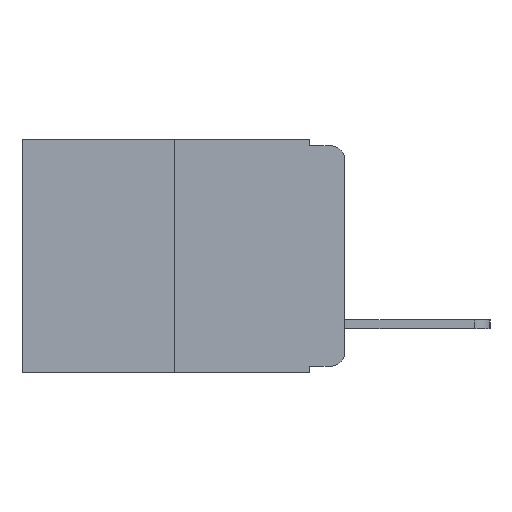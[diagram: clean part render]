
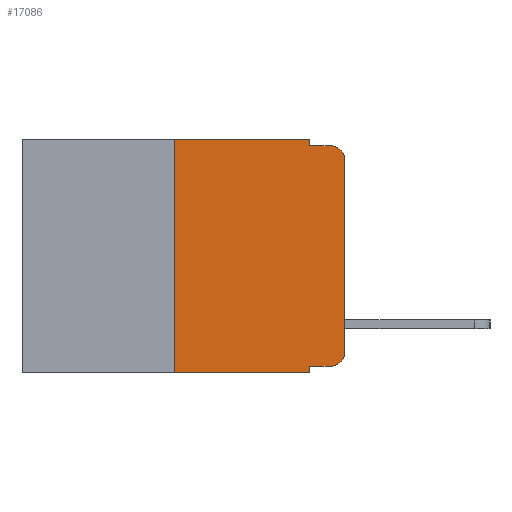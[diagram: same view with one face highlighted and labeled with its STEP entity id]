
A CAD part, left-side view. The second image highlights one B-rep face of the part: STEP entity #17086.
In plain terms, the highlighted planar face has unit normal (-1, 0, 0).
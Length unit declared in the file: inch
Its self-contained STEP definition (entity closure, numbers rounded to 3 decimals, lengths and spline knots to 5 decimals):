
#43 = DIRECTION ( 'NONE',  ( 0., 0., -1. ) ) ;
#70 = DIRECTION ( 'NONE',  ( 0., 0., -1. ) ) ;
#181 = CARTESIAN_POINT ( 'NONE',  ( 0., 0.051, -0.333 ) ) ;
#189 = CARTESIAN_POINT ( 'NONE',  ( 0., 0.051, -0.01 ) ) ;
#277 = CARTESIAN_POINT ( 'NONE',  ( 0., 0.25, 0. ) ) ;
#393 = VECTOR ( 'NONE', #15945, 39.37008 ) ;
#507 = EDGE_CURVE ( 'NONE', #2169, #3203, #17074, .T. ) ;
#1768 = EDGE_CURVE ( 'NONE', #7908, #6309, #15656, .T. ) ;
#1903 = ORIENTED_EDGE ( 'NONE', *, *, #3409, .T. ) ;
#1991 = CARTESIAN_POINT ( 'NONE',  ( 0., 0.473, 0. ) ) ;
#2058 = CIRCLE ( 'NONE', #14012, 0.02 ) ;
#2169 = VERTEX_POINT ( 'NONE', #181 ) ;
#2382 = LINE ( 'NONE', #9124, #9627 ) ;
#2797 = AXIS2_PLACEMENT_3D ( 'NONE', #1991, #3317, #12769 ) ;
#2988 = CARTESIAN_POINT ( 'NONE',  ( 0., 0.02, -0.01 ) ) ;
#3203 = VERTEX_POINT ( 'NONE', #14636 ) ;
#3317 = DIRECTION ( 'NONE',  ( 1., 0., 0. ) ) ;
#3409 = EDGE_CURVE ( 'NONE', #8566, #10342, #2058, .T. ) ;
#3443 = AXIS2_PLACEMENT_3D ( 'NONE', #16020, #8239, #70 ) ;
#3551 = ORIENTED_EDGE ( 'NONE', *, *, #12617, .T. ) ;
#3612 = CARTESIAN_POINT ( 'NONE',  ( 0., 0.051, 0. ) ) ;
#3906 = EDGE_CURVE ( 'NONE', #12647, #9530, #4733, .T. ) ;
#4061 = LINE ( 'NONE', #15354, #14318 ) ;
#4464 = CARTESIAN_POINT ( 'NONE',  ( 0., 0.02, -0.03 ) ) ;
#4733 = CIRCLE ( 'NONE', #3443, 0.02 ) ;
#5234 = EDGE_CURVE ( 'NONE', #9530, #8566, #4061, .T. ) ;
#5335 = LINE ( 'NONE', #9061, #15106 ) ;
#5355 = EDGE_CURVE ( 'NONE', #7908, #3203, #2382, .T. ) ;
#5852 = DIRECTION ( 'NONE',  ( 0., 0., -1. ) ) ;
#5907 = ORIENTED_EDGE ( 'NONE', *, *, #11733, .F. ) ;
#5993 = CARTESIAN_POINT ( 'NONE',  ( 0., 0., -0.03 ) ) ;
#6309 = VERTEX_POINT ( 'NONE', #277 ) ;
#6350 = ORIENTED_EDGE ( 'NONE', *, *, #9936, .F. ) ;
#6707 = VERTEX_POINT ( 'NONE', #9247 ) ;
#7534 = DIRECTION ( 'NONE',  ( 0., 0., 1. ) ) ;
#7908 = VERTEX_POINT ( 'NONE', #13844 ) ;
#7987 = EDGE_LOOP ( 'NONE', ( #8689, #1903, #9123, #5907, #6350, #9981, #13858, #17171, #3551, #14247 ) ) ;
#8163 = CARTESIAN_POINT ( 'NONE',  ( 0., 0.051, -0.333 ) ) ;
#8239 = DIRECTION ( 'NONE',  ( -1., 0., 0. ) ) ;
#8566 = VERTEX_POINT ( 'NONE', #5993 ) ;
#8689 = ORIENTED_EDGE ( 'NONE', *, *, #5234, .T. ) ;
#8842 = DIRECTION ( 'NONE',  ( 0., 0., 1. ) ) ;
#8938 = LINE ( 'NONE', #15477, #11660 ) ;
#9061 = CARTESIAN_POINT ( 'NONE',  ( 0., 0.473, 0. ) ) ;
#9123 = ORIENTED_EDGE ( 'NONE', *, *, #10297, .F. ) ;
#9124 = CARTESIAN_POINT ( 'NONE',  ( 0., 0.473, -0.343 ) ) ;
#9247 = CARTESIAN_POINT ( 'NONE',  ( 0., 0.051, -0.01 ) ) ;
#9419 = LINE ( 'NONE', #189, #12537 ) ;
#9530 = VERTEX_POINT ( 'NONE', #15962 ) ;
#9615 = VECTOR ( 'NONE', #8842, 39.37008 ) ;
#9627 = VECTOR ( 'NONE', #10471, 39.37008 ) ;
#9936 = EDGE_CURVE ( 'NONE', #6309, #10650, #5335, .T. ) ;
#9981 = ORIENTED_EDGE ( 'NONE', *, *, #1768, .F. ) ;
#10129 = PLANE ( 'NONE',  #2797 ) ;
#10297 = EDGE_CURVE ( 'NONE', #6707, #10342, #9419, .T. ) ;
#10330 = DIRECTION ( 'NONE',  ( 0., 0., -1. ) ) ;
#10342 = VERTEX_POINT ( 'NONE', #2988 ) ;
#10471 = DIRECTION ( 'NONE',  ( 0., -1., 0. ) ) ;
#10650 = VERTEX_POINT ( 'NONE', #3612 ) ;
#11058 = DIRECTION ( 'NONE',  ( 0., -1., 0. ) ) ;
#11149 = CARTESIAN_POINT ( 'NONE',  ( 0., 0.051, 0. ) ) ;
#11218 = LINE ( 'NONE', #8163, #393 ) ;
#11660 = VECTOR ( 'NONE', #10330, 39.37008 ) ;
#11733 = EDGE_CURVE ( 'NONE', #10650, #6707, #8938, .T. ) ;
#12208 = CARTESIAN_POINT ( 'NONE',  ( 0., 0.02, -0.333 ) ) ;
#12537 = VECTOR ( 'NONE', #11058, 39.37008 ) ;
#12617 = EDGE_CURVE ( 'NONE', #2169, #12647, #11218, .T. ) ;
#12647 = VERTEX_POINT ( 'NONE', #12208 ) ;
#12769 = DIRECTION ( 'NONE',  ( 0., 0., -1. ) ) ;
#13586 = FACE_OUTER_BOUND ( 'NONE', #7987, .T. ) ;
#13844 = CARTESIAN_POINT ( 'NONE',  ( 0., 0.25, -0.343 ) ) ;
#13858 = ORIENTED_EDGE ( 'NONE', *, *, #5355, .T. ) ;
#13866 = DIRECTION ( 'NONE',  ( -1., 0., 0. ) ) ;
#14012 = AXIS2_PLACEMENT_3D ( 'NONE', #4464, #13866, #5852 ) ;
#14154 = VECTOR ( 'NONE', #43, 39.37008 ) ;
#14247 = ORIENTED_EDGE ( 'NONE', *, *, #3906, .T. ) ;
#14318 = VECTOR ( 'NONE', #7534, 39.37008 ) ;
#14324 = DIRECTION ( 'NONE',  ( 0., -1., 0. ) ) ;
#14636 = CARTESIAN_POINT ( 'NONE',  ( 0., 0.051, -0.343 ) ) ;
#15106 = VECTOR ( 'NONE', #14324, 39.37008 ) ;
#15354 = CARTESIAN_POINT ( 'NONE',  ( 0., 0., 0. ) ) ;
#15477 = CARTESIAN_POINT ( 'NONE',  ( 0., 0.051, 0. ) ) ;
#15656 = LINE ( 'NONE', #16588, #9615 ) ;
#15945 = DIRECTION ( 'NONE',  ( 0., -1., 0. ) ) ;
#15962 = CARTESIAN_POINT ( 'NONE',  ( 0., 0., -0.313 ) ) ;
#16020 = CARTESIAN_POINT ( 'NONE',  ( 0., 0.02, -0.313 ) ) ;
#16588 = CARTESIAN_POINT ( 'NONE',  ( 0., 0.25, 0. ) ) ;
#17074 = LINE ( 'NONE', #11149, #14154 ) ;
#17086 = ADVANCED_FACE ( 'NONE', ( #13586 ), #10129, .F. ) ;
#17171 = ORIENTED_EDGE ( 'NONE', *, *, #507, .F. ) ;
